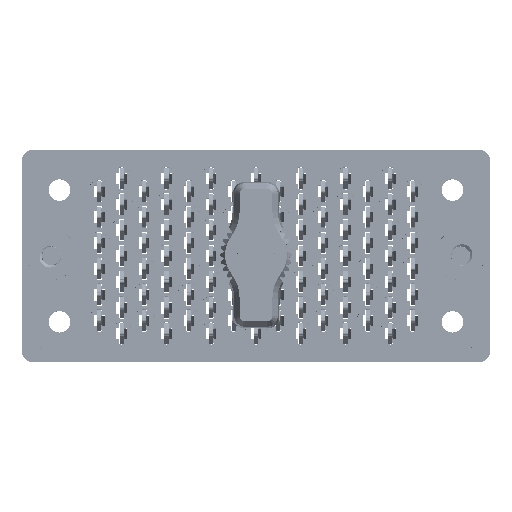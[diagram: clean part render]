
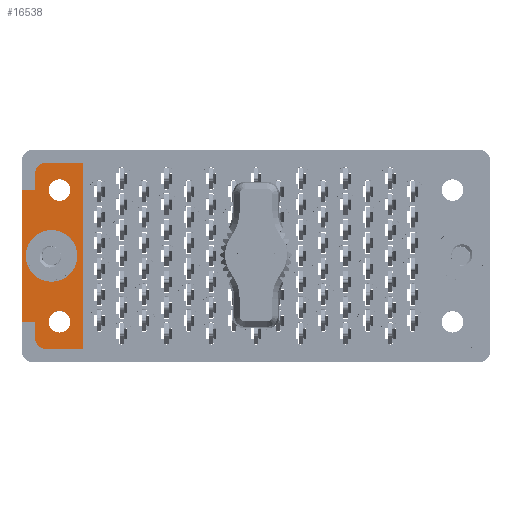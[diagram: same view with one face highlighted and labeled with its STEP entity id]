
A CAD part, top view. The second image highlights one B-rep face of the part: STEP entity #16538.
In plain terms, the highlighted planar face has unit normal (0, 0, 1).
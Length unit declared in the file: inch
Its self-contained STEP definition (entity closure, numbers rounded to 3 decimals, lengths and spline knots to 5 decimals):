
#693 = ORIENTED_EDGE ( 'NONE', *, *, #72677, .F. ) ;
#1377 = ORIENTED_EDGE ( 'NONE', *, *, #11853, .T. ) ;
#4822 = VERTEX_POINT ( 'NONE', #76241 ) ;
#5124 = ORIENTED_EDGE ( 'NONE', *, *, #6338, .F. ) ;
#5150 = AXIS2_PLACEMENT_3D ( 'NONE', #91820, #10297, #62471 ) ;
#5328 = CARTESIAN_POINT ( 'NONE',  ( -1.2825, 0., -0.117 ) ) ;
#5865 = EDGE_CURVE ( 'NONE', #4822, #85605, #41373, .T. ) ;
#6338 = EDGE_CURVE ( 'NONE', #85605, #4822, #35456, .T. ) ;
#6469 = VECTOR ( 'NONE', #57502, 39.37008 ) ;
#9242 = CARTESIAN_POINT ( 'NONE',  ( -1.141, -0.3825, -0.117 ) ) ;
#9409 = AXIS2_PLACEMENT_3D ( 'NONE', #9242, #81919, #37181 ) ;
#9526 = CARTESIAN_POINT ( 'NONE',  ( -1.2825, -0.478, -0.117 ) ) ;
#10297 = DIRECTION ( 'NONE',  ( 0., 0., 1. ) ) ;
#10369 = AXIS2_PLACEMENT_3D ( 'NONE', #54279, #91482, #46743 ) ;
#11752 = CARTESIAN_POINT ( 'NONE',  ( -1.2205, -0.54, -0.117 ) ) ;
#11853 = EDGE_CURVE ( 'NONE', #29073, #26804, #66211, .T. ) ;
#12542 = CARTESIAN_POINT ( 'NONE',  ( -1.1875, 0., -0.117 ) ) ;
#14402 = ORIENTED_EDGE ( 'NONE', *, *, #39354, .T. ) ;
#14752 = DIRECTION ( 'NONE',  ( -1., 0., 0. ) ) ;
#16097 = VECTOR ( 'NONE', #14752, 39.37008 ) ;
#16538 = ADVANCED_FACE ( 'NONE', ( #82462, #34581, #32281, #75478 ), #62206, .T. ) ;
#17259 = CARTESIAN_POINT ( 'NONE',  ( -1.359, 0.617, -0.117 ) ) ;
#18843 = EDGE_LOOP ( 'NONE', ( #48182, #91610 ) ) ;
#20407 = ORIENTED_EDGE ( 'NONE', *, *, #29442, .T. ) ;
#20674 = DIRECTION ( 'NONE',  ( 1., 0., 0. ) ) ;
#21331 = LINE ( 'NONE', #48040, #96007 ) ;
#21417 = EDGE_CURVE ( 'NONE', #91238, #82489, #59804, .T. ) ;
#22991 = CARTESIAN_POINT ( 'NONE',  ( -1.0785, 0.3825, -0.117 ) ) ;
#23211 = VERTEX_POINT ( 'NONE', #52487 ) ;
#23885 = CARTESIAN_POINT ( 'NONE',  ( -1.2205, 0.478, -0.117 ) ) ;
#23948 = LINE ( 'NONE', #5328, #6469 ) ;
#24356 = CARTESIAN_POINT ( 'NONE',  ( -1.359, -0.617, -0.117 ) ) ;
#25252 = CARTESIAN_POINT ( 'NONE',  ( 0., -0.3825, -0.117 ) ) ;
#25415 = ORIENTED_EDGE ( 'NONE', *, *, #36386, .T. ) ;
#26212 = DIRECTION ( 'NONE',  ( 0., 1., 0. ) ) ;
#26631 = CARTESIAN_POINT ( 'NONE',  ( -1.2825, 0.3825, -0.117 ) ) ;
#26775 = CARTESIAN_POINT ( 'NONE',  ( 0., 0.3825, -0.117 ) ) ;
#26804 = VERTEX_POINT ( 'NONE', #41662 ) ;
#27878 = EDGE_CURVE ( 'NONE', #26804, #42877, #23948, .T. ) ;
#28515 = AXIS2_PLACEMENT_3D ( 'NONE', #23885, #38871, #76108 ) ;
#29073 = VERTEX_POINT ( 'NONE', #44511 ) ;
#29312 = DIRECTION ( 'NONE',  ( 1., 0., 0. ) ) ;
#29434 = VECTOR ( 'NONE', #78983, 39.37008 ) ;
#29442 = EDGE_CURVE ( 'NONE', #34725, #44871, #21331, .T. ) ;
#29865 = DIRECTION ( 'NONE',  ( 0., -1., 0. ) ) ;
#30952 = CARTESIAN_POINT ( 'NONE',  ( -1.359, -0.3825, -0.117 ) ) ;
#31884 = CIRCLE ( 'NONE', #5150, 0.062 ) ;
#32011 = VERTEX_POINT ( 'NONE', #9526 ) ;
#32281 = FACE_BOUND ( 'NONE', #18843, .T. ) ;
#33044 = CIRCLE ( 'NONE', #10369, 0.15 ) ;
#34581 = FACE_BOUND ( 'NONE', #70531, .T. ) ;
#34725 = VERTEX_POINT ( 'NONE', #83429 ) ;
#35456 = CIRCLE ( 'NONE', #86206, 0.0625 ) ;
#35581 = VERTEX_POINT ( 'NONE', #11752 ) ;
#36386 = EDGE_CURVE ( 'NONE', #23211, #32011, #61472, .T. ) ;
#36456 = ORIENTED_EDGE ( 'NONE', *, *, #5865, .F. ) ;
#37181 = DIRECTION ( 'NONE',  ( 1., 0., 0. ) ) ;
#37265 = LINE ( 'NONE', #17259, #69932 ) ;
#37344 = CARTESIAN_POINT ( 'NONE',  ( -1.2825, 0., -0.117 ) ) ;
#37758 = CARTESIAN_POINT ( 'NONE',  ( -1.141, 0.3825, -0.117 ) ) ;
#38081 = VERTEX_POINT ( 'NONE', #80761 ) ;
#38291 = ORIENTED_EDGE ( 'NONE', *, *, #49499, .T. ) ;
#38539 = EDGE_CURVE ( 'NONE', #32011, #35581, #31884, .T. ) ;
#38871 = DIRECTION ( 'NONE',  ( 0., 0., 1. ) ) ;
#39354 = EDGE_CURVE ( 'NONE', #42877, #55116, #69117, .T. ) ;
#39877 = ORIENTED_EDGE ( 'NONE', *, *, #79242, .T. ) ;
#41373 = CIRCLE ( 'NONE', #9409, 0.0625 ) ;
#41662 = CARTESIAN_POINT ( 'NONE',  ( -1.2825, 0.478, -0.117 ) ) ;
#42706 = VERTEX_POINT ( 'NONE', #30952 ) ;
#42855 = DIRECTION ( 'NONE',  ( 0., 0., 1. ) ) ;
#42877 = VERTEX_POINT ( 'NONE', #26631 ) ;
#43594 = AXIS2_PLACEMENT_3D ( 'NONE', #24356, #91562, #76569 ) ;
#44511 = CARTESIAN_POINT ( 'NONE',  ( -1.2205, 0.54, -0.117 ) ) ;
#44871 = VERTEX_POINT ( 'NONE', #58715 ) ;
#45029 = VECTOR ( 'NONE', #29865, 39.37008 ) ;
#45370 = ORIENTED_EDGE ( 'NONE', *, *, #27878, .T. ) ;
#46697 = VERTEX_POINT ( 'NONE', #79972 ) ;
#46743 = DIRECTION ( 'NONE',  ( 1., 0., 0. ) ) ;
#47037 = VECTOR ( 'NONE', #87845, 39.37008 ) ;
#47628 = CARTESIAN_POINT ( 'NONE',  ( -1.141, -0.3825, -0.117 ) ) ;
#48040 = CARTESIAN_POINT ( 'NONE',  ( -1.005, 0.617, -0.117 ) ) ;
#48182 = ORIENTED_EDGE ( 'NONE', *, *, #96663, .F. ) ;
#48676 = DIRECTION ( 'NONE',  ( -1., 0., 0. ) ) ;
#49499 = EDGE_CURVE ( 'NONE', #44871, #29073, #55709, .T. ) ;
#51052 = DIRECTION ( 'NONE',  ( 0., 0., 1. ) ) ;
#51870 = CARTESIAN_POINT ( 'NONE',  ( 0., 0.54, -0.117 ) ) ;
#52487 = CARTESIAN_POINT ( 'NONE',  ( -1.2825, -0.3825, -0.117 ) ) ;
#54279 = CARTESIAN_POINT ( 'NONE',  ( -1.1875, 0., -0.117 ) ) ;
#55052 = LINE ( 'NONE', #25252, #58628 ) ;
#55116 = VERTEX_POINT ( 'NONE', #74987 ) ;
#55709 = LINE ( 'NONE', #51870, #16097 ) ;
#57502 = DIRECTION ( 'NONE',  ( 0., -1., 0. ) ) ;
#58050 = CARTESIAN_POINT ( 'NONE',  ( -1.2035, 0.3825, -0.117 ) ) ;
#58628 = VECTOR ( 'NONE', #48676, 39.37008 ) ;
#58715 = CARTESIAN_POINT ( 'NONE',  ( -1.005, 0.54, -0.117 ) ) ;
#59804 = CIRCLE ( 'NONE', #60231, 0.0625 ) ;
#59965 = AXIS2_PLACEMENT_3D ( 'NONE', #12542, #42855, #20674 ) ;
#60231 = AXIS2_PLACEMENT_3D ( 'NONE', #95751, #51052, #81077 ) ;
#61472 = LINE ( 'NONE', #37344, #45029 ) ;
#62206 = PLANE ( 'NONE',  #43594 ) ;
#62471 = DIRECTION ( 'NONE',  ( 1., 0., 0. ) ) ;
#64532 = EDGE_LOOP ( 'NONE', ( #5124, #36456 ) ) ;
#65337 = CARTESIAN_POINT ( 'NONE',  ( 0., -0.54, -0.117 ) ) ;
#66211 = CIRCLE ( 'NONE', #28515, 0.062 ) ;
#66921 = LINE ( 'NONE', #65337, #47037 ) ;
#66942 = CIRCLE ( 'NONE', #78203, 0.0625 ) ;
#67145 = DIRECTION ( 'NONE',  ( 0., 0., 1. ) ) ;
#69117 = LINE ( 'NONE', #26775, #29434 ) ;
#69521 = DIRECTION ( 'NONE',  ( 1., 0., 0. ) ) ;
#69932 = VECTOR ( 'NONE', #90651, 39.37008 ) ;
#70531 = EDGE_LOOP ( 'NONE', ( #75486, #693 ) ) ;
#72677 = EDGE_CURVE ( 'NONE', #82489, #91238, #66942, .T. ) ;
#74119 = EDGE_CURVE ( 'NONE', #23211, #42706, #55052, .T. ) ;
#74987 = CARTESIAN_POINT ( 'NONE',  ( -1.359, 0.3825, -0.117 ) ) ;
#75478 = FACE_OUTER_BOUND ( 'NONE', #85593, .T. ) ;
#75486 = ORIENTED_EDGE ( 'NONE', *, *, #21417, .F. ) ;
#76108 = DIRECTION ( 'NONE',  ( 1., 0., 0. ) ) ;
#76241 = CARTESIAN_POINT ( 'NONE',  ( -1.0785, -0.3825, -0.117 ) ) ;
#76442 = DIRECTION ( 'NONE',  ( 0., 0., 1. ) ) ;
#76569 = DIRECTION ( 'NONE',  ( 1., 0., 0. ) ) ;
#78203 = AXIS2_PLACEMENT_3D ( 'NONE', #37758, #67145, #29312 ) ;
#78983 = DIRECTION ( 'NONE',  ( -1., 0., 0. ) ) ;
#79242 = EDGE_CURVE ( 'NONE', #55116, #42706, #37265, .T. ) ;
#79972 = CARTESIAN_POINT ( 'NONE',  ( -1.0375, 0., -0.117 ) ) ;
#80056 = CIRCLE ( 'NONE', #59965, 0.15 ) ;
#80761 = CARTESIAN_POINT ( 'NONE',  ( -1.3375, 0., -0.117 ) ) ;
#81077 = DIRECTION ( 'NONE',  ( 1., 0., 0. ) ) ;
#81919 = DIRECTION ( 'NONE',  ( 0., 0., 1. ) ) ;
#82462 = FACE_BOUND ( 'NONE', #64532, .T. ) ;
#82489 = VERTEX_POINT ( 'NONE', #22991 ) ;
#83429 = CARTESIAN_POINT ( 'NONE',  ( -1.005, -0.54, -0.117 ) ) ;
#84734 = EDGE_CURVE ( 'NONE', #34725, #35581, #66921, .T. ) ;
#84804 = CARTESIAN_POINT ( 'NONE',  ( -1.2035, -0.3825, -0.117 ) ) ;
#85593 = EDGE_LOOP ( 'NONE', ( #25415, #89050, #88926, #20407, #38291, #1377, #45370, #14402, #39877, #85858 ) ) ;
#85605 = VERTEX_POINT ( 'NONE', #84804 ) ;
#85858 = ORIENTED_EDGE ( 'NONE', *, *, #74119, .F. ) ;
#86206 = AXIS2_PLACEMENT_3D ( 'NONE', #47628, #76442, #69521 ) ;
#87845 = DIRECTION ( 'NONE',  ( -1., 0., 0. ) ) ;
#88926 = ORIENTED_EDGE ( 'NONE', *, *, #84734, .F. ) ;
#89050 = ORIENTED_EDGE ( 'NONE', *, *, #38539, .T. ) ;
#89551 = EDGE_CURVE ( 'NONE', #38081, #46697, #80056, .T. ) ;
#90651 = DIRECTION ( 'NONE',  ( 0., -1., 0. ) ) ;
#91238 = VERTEX_POINT ( 'NONE', #58050 ) ;
#91482 = DIRECTION ( 'NONE',  ( 0., 0., 1. ) ) ;
#91562 = DIRECTION ( 'NONE',  ( 0., 0., 1. ) ) ;
#91610 = ORIENTED_EDGE ( 'NONE', *, *, #89551, .F. ) ;
#91820 = CARTESIAN_POINT ( 'NONE',  ( -1.2205, -0.478, -0.117 ) ) ;
#95751 = CARTESIAN_POINT ( 'NONE',  ( -1.141, 0.3825, -0.117 ) ) ;
#96007 = VECTOR ( 'NONE', #26212, 39.37008 ) ;
#96663 = EDGE_CURVE ( 'NONE', #46697, #38081, #33044, .T. ) ;
